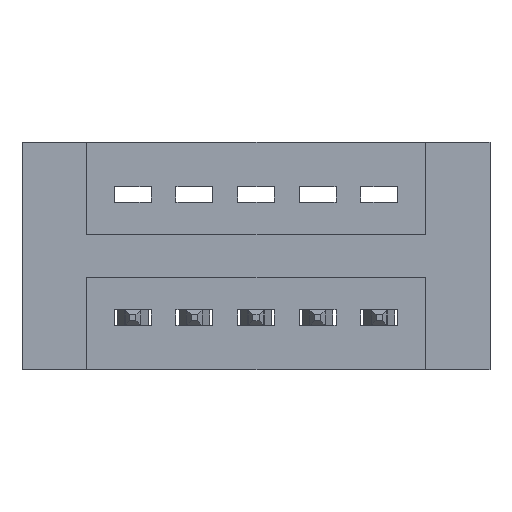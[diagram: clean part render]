
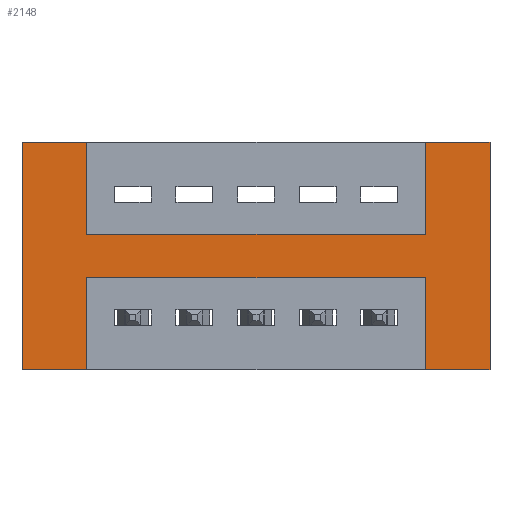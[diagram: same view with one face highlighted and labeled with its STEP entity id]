
A CAD part, front view. The second image highlights one B-rep face of the part: STEP entity #2148.
In plain terms, the highlighted planar face has unit normal (0, -1, 0).
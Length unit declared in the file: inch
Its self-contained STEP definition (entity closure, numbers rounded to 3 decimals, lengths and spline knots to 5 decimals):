
#8 = ORIENTED_EDGE ( 'NONE', *, *, #3031, .F. ) ;
#14 = ORIENTED_EDGE ( 'NONE', *, *, #6849, .T. ) ;
#557 = VECTOR ( 'NONE', #8067, 39.37008 ) ;
#605 = DIRECTION ( 'NONE',  ( 1., 0., 0. ) ) ;
#656 = VERTEX_POINT ( 'NONE', #6973 ) ;
#746 = VERTEX_POINT ( 'NONE', #3816 ) ;
#826 = DIRECTION ( 'NONE',  ( -1., 0., 0. ) ) ;
#1116 = LINE ( 'NONE', #1343, #3761 ) ;
#1126 = LINE ( 'NONE', #6184, #4385 ) ;
#1276 = CARTESIAN_POINT ( 'NONE',  ( 0., 0., -0.37 ) ) ;
#1302 = VECTOR ( 'NONE', #7198, 39.37008 ) ;
#1313 = EDGE_LOOP ( 'NONE', ( #14, #2219, #1353, #2672, #4480, #4516, #6426, #4576, #4454, #7458, #3466, #8 ) ) ;
#1319 = VERTEX_POINT ( 'NONE', #5417 ) ;
#1343 = CARTESIAN_POINT ( 'NONE',  ( 0.3925, 0., -0.22 ) ) ;
#1353 = ORIENTED_EDGE ( 'NONE', *, *, #7553, .F. ) ;
#1434 = VECTOR ( 'NONE', #605, 39.37008 ) ;
#1465 = CARTESIAN_POINT ( 'NONE',  ( 0., 0., -0.37 ) ) ;
#1485 = AXIS2_PLACEMENT_3D ( 'NONE', #1276, #5198, #7796 ) ;
#1496 = CARTESIAN_POINT ( 'NONE',  ( 0.2875, 0., 0. ) ) ;
#1511 = EDGE_CURVE ( 'NONE', #1803, #656, #4819, .T. ) ;
#1516 = LINE ( 'NONE', #5440, #4776 ) ;
#1644 = LINE ( 'NONE', #7717, #1434 ) ;
#1746 = CARTESIAN_POINT ( 'NONE',  ( 0.9425, 0., 0. ) ) ;
#1765 = VECTOR ( 'NONE', #4929, 39.37008 ) ;
#1803 = VERTEX_POINT ( 'NONE', #1496 ) ;
#1817 = VECTOR ( 'NONE', #6208, 39.37008 ) ;
#1857 = EDGE_CURVE ( 'NONE', #4812, #3729, #3989, .T. ) ;
#2148 = ADVANCED_FACE ( 'NONE', ( #2345 ), #5897, .T. ) ;
#2219 = ORIENTED_EDGE ( 'NONE', *, *, #1857, .F. ) ;
#2268 = CARTESIAN_POINT ( 'NONE',  ( 0.9425, 0., 0. ) ) ;
#2312 = CARTESIAN_POINT ( 'NONE',  ( 0.2875, 0., 0. ) ) ;
#2334 = CARTESIAN_POINT ( 'NONE',  ( 0., 0., -0.37 ) ) ;
#2345 = FACE_OUTER_BOUND ( 'NONE', #1313, .T. ) ;
#2501 = LINE ( 'NONE', #6489, #1302 ) ;
#2535 = DIRECTION ( 'NONE',  ( 0., 0., 1. ) ) ;
#2672 = ORIENTED_EDGE ( 'NONE', *, *, #7199, .F. ) ;
#2719 = EDGE_CURVE ( 'NONE', #1803, #4930, #1644, .T. ) ;
#3031 = EDGE_CURVE ( 'NONE', #746, #3607, #3873, .T. ) ;
#3445 = EDGE_CURVE ( 'NONE', #4544, #1319, #1116, .T. ) ;
#3466 = ORIENTED_EDGE ( 'NONE', *, *, #5272, .F. ) ;
#3598 = DIRECTION ( 'NONE',  ( 0., 0., -1. ) ) ;
#3607 = VERTEX_POINT ( 'NONE', #4721 ) ;
#3729 = VERTEX_POINT ( 'NONE', #6393 ) ;
#3761 = VECTOR ( 'NONE', #6545, 39.37008 ) ;
#3816 = CARTESIAN_POINT ( 'NONE',  ( 1.0475, 0., -0.37 ) ) ;
#3873 = LINE ( 'NONE', #2334, #7582 ) ;
#3989 = LINE ( 'NONE', #8202, #1765 ) ;
#4112 = DIRECTION ( 'NONE',  ( 0., 0., 1. ) ) ;
#4385 = VECTOR ( 'NONE', #4112, 39.37008 ) ;
#4454 = ORIENTED_EDGE ( 'NONE', *, *, #7859, .F. ) ;
#4480 = ORIENTED_EDGE ( 'NONE', *, *, #5901, .F. ) ;
#4516 = ORIENTED_EDGE ( 'NONE', *, *, #2719, .F. ) ;
#4544 = VERTEX_POINT ( 'NONE', #4697 ) ;
#4576 = ORIENTED_EDGE ( 'NONE', *, *, #5870, .F. ) ;
#4697 = CARTESIAN_POINT ( 'NONE',  ( 0.9425, 0., -0.22 ) ) ;
#4721 = CARTESIAN_POINT ( 'NONE',  ( 0.9425, 0., -0.37 ) ) ;
#4724 = CARTESIAN_POINT ( 'NONE',  ( 0.3925, 0., -0.15 ) ) ;
#4776 = VECTOR ( 'NONE', #3598, 39.37008 ) ;
#4812 = VERTEX_POINT ( 'NONE', #1746 ) ;
#4819 = LINE ( 'NONE', #2312, #8011 ) ;
#4929 = DIRECTION ( 'NONE',  ( 1., 0., 0. ) ) ;
#4930 = VERTEX_POINT ( 'NONE', #5552 ) ;
#4994 = LINE ( 'NONE', #1465, #8494 ) ;
#5147 = LINE ( 'NONE', #8165, #557 ) ;
#5198 = DIRECTION ( 'NONE',  ( 0., -1., 0. ) ) ;
#5255 = LINE ( 'NONE', #2268, #6392 ) ;
#5272 = EDGE_CURVE ( 'NONE', #3607, #4544, #1126, .T. ) ;
#5366 = LINE ( 'NONE', #8129, #1817 ) ;
#5417 = CARTESIAN_POINT ( 'NONE',  ( 0.3925, 0., -0.22 ) ) ;
#5440 = CARTESIAN_POINT ( 'NONE',  ( 0.3925, 0., 0. ) ) ;
#5552 = CARTESIAN_POINT ( 'NONE',  ( 0.3925, 0., 0. ) ) ;
#5870 = EDGE_CURVE ( 'NONE', #7066, #656, #4994, .T. ) ;
#5897 = PLANE ( 'NONE',  #1485 ) ;
#5901 = EDGE_CURVE ( 'NONE', #4930, #7350, #1516, .T. ) ;
#5962 = CARTESIAN_POINT ( 'NONE',  ( 0.9425, 0., -0.15 ) ) ;
#6184 = CARTESIAN_POINT ( 'NONE',  ( 0.9425, 0., -0.37 ) ) ;
#6208 = DIRECTION ( 'NONE',  ( 0., 0., 1. ) ) ;
#6392 = VECTOR ( 'NONE', #2535, 39.37008 ) ;
#6393 = CARTESIAN_POINT ( 'NONE',  ( 1.0475, 0., 0. ) ) ;
#6426 = ORIENTED_EDGE ( 'NONE', *, *, #1511, .T. ) ;
#6489 = CARTESIAN_POINT ( 'NONE',  ( 0.3925, 0., -0.15 ) ) ;
#6545 = DIRECTION ( 'NONE',  ( -1., 0., 0. ) ) ;
#6849 = EDGE_CURVE ( 'NONE', #746, #3729, #5366, .T. ) ;
#6973 = CARTESIAN_POINT ( 'NONE',  ( 0.2875, 0., -0.37 ) ) ;
#7066 = VERTEX_POINT ( 'NONE', #7068 ) ;
#7068 = CARTESIAN_POINT ( 'NONE',  ( 0.3925, 0., -0.37 ) ) ;
#7198 = DIRECTION ( 'NONE',  ( 1., 0., 0. ) ) ;
#7199 = EDGE_CURVE ( 'NONE', #7350, #8187, #2501, .T. ) ;
#7350 = VERTEX_POINT ( 'NONE', #4724 ) ;
#7432 = DIRECTION ( 'NONE',  ( -1., 0., 0. ) ) ;
#7458 = ORIENTED_EDGE ( 'NONE', *, *, #3445, .F. ) ;
#7553 = EDGE_CURVE ( 'NONE', #8187, #4812, #5255, .T. ) ;
#7582 = VECTOR ( 'NONE', #7432, 39.37008 ) ;
#7717 = CARTESIAN_POINT ( 'NONE',  ( 0., 0., 0. ) ) ;
#7796 = DIRECTION ( 'NONE',  ( 0., 0., -1. ) ) ;
#7859 = EDGE_CURVE ( 'NONE', #1319, #7066, #5147, .T. ) ;
#8011 = VECTOR ( 'NONE', #8377, 39.37008 ) ;
#8067 = DIRECTION ( 'NONE',  ( 0., 0., -1. ) ) ;
#8129 = CARTESIAN_POINT ( 'NONE',  ( 1.0475, 0., 0. ) ) ;
#8165 = CARTESIAN_POINT ( 'NONE',  ( 0.3925, 0., -0.37 ) ) ;
#8187 = VERTEX_POINT ( 'NONE', #5962 ) ;
#8202 = CARTESIAN_POINT ( 'NONE',  ( 0., 0., 0. ) ) ;
#8377 = DIRECTION ( 'NONE',  ( 0., 0., -1. ) ) ;
#8494 = VECTOR ( 'NONE', #826, 39.37008 ) ;
